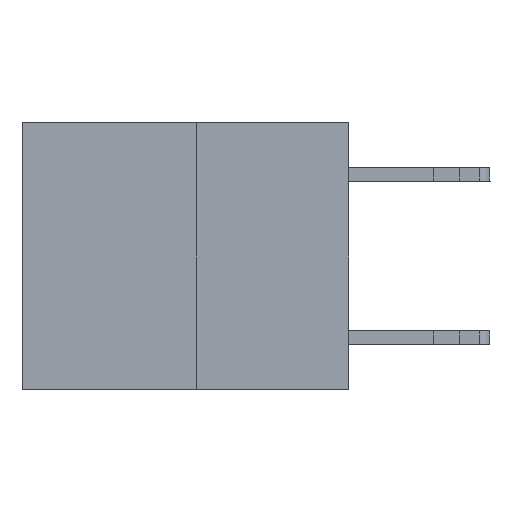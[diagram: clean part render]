
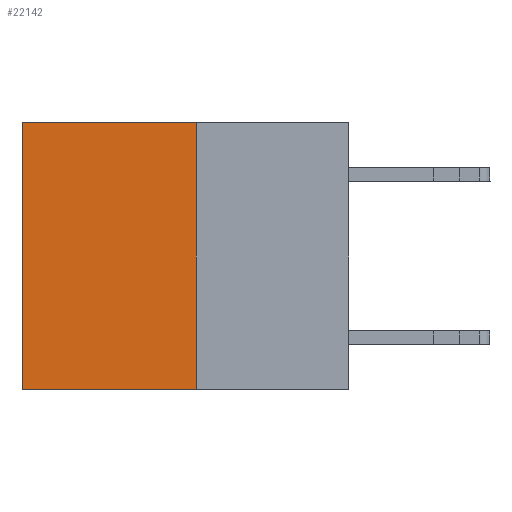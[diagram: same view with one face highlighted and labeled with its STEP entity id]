
A CAD part, left-side view. The second image highlights one B-rep face of the part: STEP entity #22142.
In plain terms, the highlighted planar face has unit normal (-1, 0, 0).
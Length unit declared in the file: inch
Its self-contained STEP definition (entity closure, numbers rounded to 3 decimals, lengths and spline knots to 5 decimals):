
#266 = DIRECTION ( 'NONE',  ( 0., 1., 0. ) ) ;
#460 = EDGE_LOOP ( 'NONE', ( #24005, #15662, #25842, #2943 ) ) ;
#1404 = CARTESIAN_POINT ( 'NONE',  ( 0.3165, 0.28, -0.49 ) ) ;
#1725 = VERTEX_POINT ( 'NONE', #30049 ) ;
#1900 = DIRECTION ( 'NONE',  ( 0., 0., -1. ) ) ;
#2824 = VECTOR ( 'NONE', #1900, 39.37008 ) ;
#2943 = ORIENTED_EDGE ( 'NONE', *, *, #25699, .T. ) ;
#3343 = CARTESIAN_POINT ( 'NONE',  ( 0.3165, 0.6, -0.49 ) ) ;
#3657 = VERTEX_POINT ( 'NONE', #22135 ) ;
#4782 = DIRECTION ( 'NONE',  ( 0., 0., -1. ) ) ;
#4885 = EDGE_CURVE ( 'NONE', #3657, #20159, #21372, .T. ) ;
#5083 = CARTESIAN_POINT ( 'NONE',  ( 0.3165, 0.28, -0.49 ) ) ;
#6730 = LINE ( 'NONE', #24454, #8906 ) ;
#8245 = CARTESIAN_POINT ( 'NONE',  ( 0.3165, 0.28, -0.49 ) ) ;
#8906 = VECTOR ( 'NONE', #26792, 39.37008 ) ;
#9024 = LINE ( 'NONE', #29584, #2824 ) ;
#9445 = LINE ( 'NONE', #5083, #20286 ) ;
#11830 = FACE_OUTER_BOUND ( 'NONE', #460, .T. ) ;
#13069 = DIRECTION ( 'NONE',  ( 0., 0., -1. ) ) ;
#14856 = VECTOR ( 'NONE', #4782, 39.37008 ) ;
#15378 = EDGE_CURVE ( 'NONE', #20159, #18484, #9445, .T. ) ;
#15662 = ORIENTED_EDGE ( 'NONE', *, *, #15378, .F. ) ;
#16319 = CARTESIAN_POINT ( 'NONE',  ( 0.3165, 0.28, -0.49 ) ) ;
#18484 = VERTEX_POINT ( 'NONE', #3343 ) ;
#20159 = VERTEX_POINT ( 'NONE', #8245 ) ;
#20162 = PLANE ( 'NONE',  #21663 ) ;
#20286 = VECTOR ( 'NONE', #266, 39.37008 ) ;
#21372 = LINE ( 'NONE', #16319, #14856 ) ;
#21663 = AXIS2_PLACEMENT_3D ( 'NONE', #1404, #22383, #13069 ) ;
#22135 = CARTESIAN_POINT ( 'NONE',  ( 0.3165, 0.28, 0. ) ) ;
#22142 = ADVANCED_FACE ( 'NONE', ( #11830 ), #20162, .F. ) ;
#22383 = DIRECTION ( 'NONE',  ( 1., 0., 0. ) ) ;
#24005 = ORIENTED_EDGE ( 'NONE', *, *, #24199, .T. ) ;
#24199 = EDGE_CURVE ( 'NONE', #1725, #18484, #9024, .T. ) ;
#24454 = CARTESIAN_POINT ( 'NONE',  ( 0.3165, 0.28, 0. ) ) ;
#25699 = EDGE_CURVE ( 'NONE', #3657, #1725, #6730, .T. ) ;
#25842 = ORIENTED_EDGE ( 'NONE', *, *, #4885, .F. ) ;
#26792 = DIRECTION ( 'NONE',  ( 0., 1., 0. ) ) ;
#29584 = CARTESIAN_POINT ( 'NONE',  ( 0.3165, 0.6, -0.49 ) ) ;
#30049 = CARTESIAN_POINT ( 'NONE',  ( 0.3165, 0.6, 0. ) ) ;
